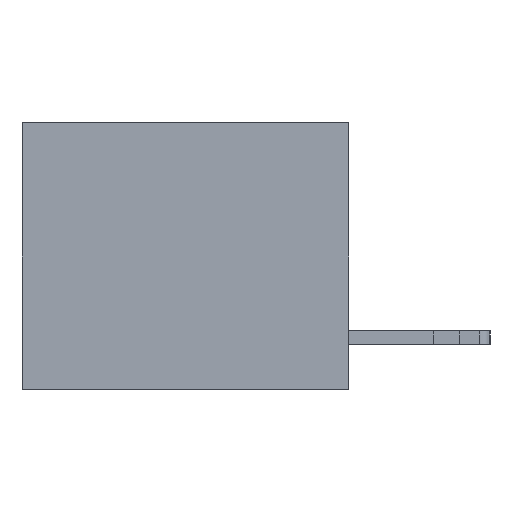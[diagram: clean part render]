
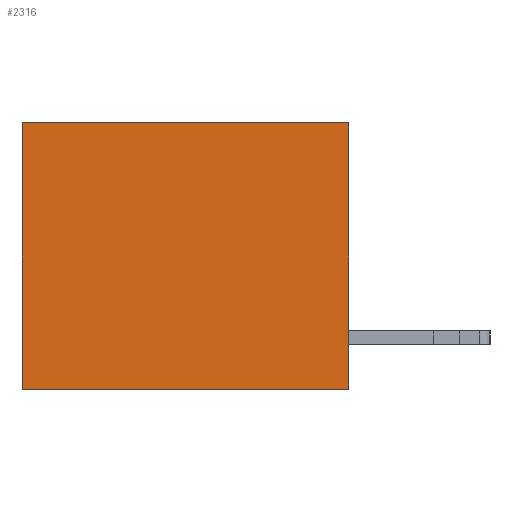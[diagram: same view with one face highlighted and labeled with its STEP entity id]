
A CAD part, left-side view. The second image highlights one B-rep face of the part: STEP entity #2316.
In plain terms, the highlighted planar face has unit normal (-1, 0, 0).
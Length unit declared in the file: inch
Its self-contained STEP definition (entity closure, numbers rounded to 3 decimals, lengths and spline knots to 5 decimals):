
#149 = DIRECTION ( 'NONE',  ( 0., 0., -1. ) ) ;
#232 = VECTOR ( 'NONE', #3802, 39.37008 ) ;
#256 = ORIENTED_EDGE ( 'NONE', *, *, #9311, .F. ) ;
#311 = ORIENTED_EDGE ( 'NONE', *, *, #11774, .T. ) ;
#314 = DIRECTION ( 'NONE',  ( 0., 1., 0. ) ) ;
#343 = EDGE_CURVE ( 'NONE', #13433, #9199, #14877, .T. ) ;
#381 = ORIENTED_EDGE ( 'NONE', *, *, #1640, .T. ) ;
#1324 = CARTESIAN_POINT ( 'NONE',  ( 0.3165, 0., -0.49 ) ) ;
#1640 = EDGE_CURVE ( 'NONE', #8573, #4344, #3569, .T. ) ;
#1677 = VECTOR ( 'NONE', #314, 39.37008 ) ;
#2316 = ADVANCED_FACE ( 'NONE', ( #6487 ), #7110, .F. ) ;
#2729 = CARTESIAN_POINT ( 'NONE',  ( 0.3165, 0.6, 0. ) ) ;
#2992 = VECTOR ( 'NONE', #4663, 39.37008 ) ;
#3569 = LINE ( 'NONE', #3762, #232 ) ;
#3688 = CARTESIAN_POINT ( 'NONE',  ( 0.3165, 0., 0. ) ) ;
#3762 = CARTESIAN_POINT ( 'NONE',  ( 0.3165, 0., 0. ) ) ;
#3802 = DIRECTION ( 'NONE',  ( 0., 1., 0. ) ) ;
#4273 = ORIENTED_EDGE ( 'NONE', *, *, #343, .F. ) ;
#4344 = VERTEX_POINT ( 'NONE', #2729 ) ;
#4630 = DIRECTION ( 'NONE',  ( 1., 0., 0. ) ) ;
#4663 = DIRECTION ( 'NONE',  ( 0., 0., -1. ) ) ;
#5617 = AXIS2_PLACEMENT_3D ( 'NONE', #11808, #4630, #9252 ) ;
#6487 = FACE_OUTER_BOUND ( 'NONE', #14353, .T. ) ;
#7110 = PLANE ( 'NONE',  #5617 ) ;
#8573 = VERTEX_POINT ( 'NONE', #3688 ) ;
#9133 = CARTESIAN_POINT ( 'NONE',  ( 0.3165, 0.6, -0.49 ) ) ;
#9199 = VERTEX_POINT ( 'NONE', #14600 ) ;
#9252 = DIRECTION ( 'NONE',  ( 0., 0., -1. ) ) ;
#9311 = EDGE_CURVE ( 'NONE', #8573, #13433, #9934, .T. ) ;
#9934 = LINE ( 'NONE', #14066, #2992 ) ;
#10928 = LINE ( 'NONE', #9133, #12226 ) ;
#11774 = EDGE_CURVE ( 'NONE', #4344, #9199, #10928, .T. ) ;
#11808 = CARTESIAN_POINT ( 'NONE',  ( 0.3165, 0., -0.49 ) ) ;
#12226 = VECTOR ( 'NONE', #149, 39.37008 ) ;
#12793 = CARTESIAN_POINT ( 'NONE',  ( 0.3165, 0., -0.49 ) ) ;
#13433 = VERTEX_POINT ( 'NONE', #12793 ) ;
#14066 = CARTESIAN_POINT ( 'NONE',  ( 0.3165, 0., -0.49 ) ) ;
#14353 = EDGE_LOOP ( 'NONE', ( #311, #4273, #256, #381 ) ) ;
#14600 = CARTESIAN_POINT ( 'NONE',  ( 0.3165, 0.6, -0.49 ) ) ;
#14877 = LINE ( 'NONE', #1324, #1677 ) ;
